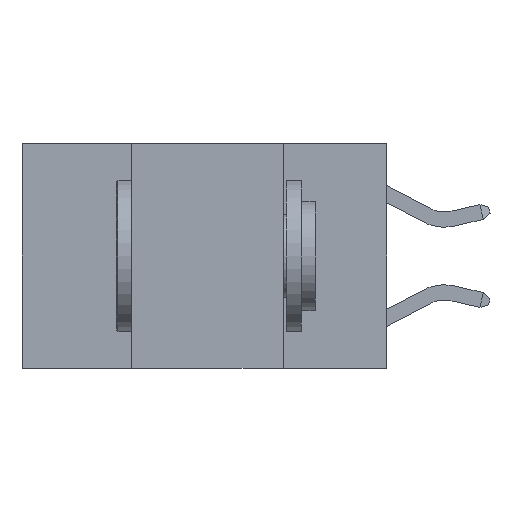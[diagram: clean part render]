
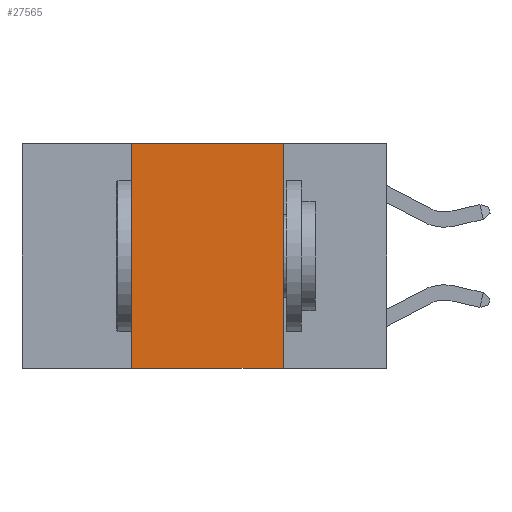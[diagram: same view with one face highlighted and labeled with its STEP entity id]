
A CAD part, left-side view. The second image highlights one B-rep face of the part: STEP entity #27565.
In plain terms, the highlighted planar face has unit normal (-1, 0, 0).
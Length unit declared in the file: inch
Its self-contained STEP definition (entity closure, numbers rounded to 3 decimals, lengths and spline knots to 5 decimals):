
#83 = ORIENTED_EDGE ( 'NONE', *, *, #22307, .F. ) ;
#902 = CARTESIAN_POINT ( 'NONE',  ( 0., 0.6, 0. ) ) ;
#1982 = LINE ( 'NONE', #8722, #28804 ) ;
#2280 = ORIENTED_EDGE ( 'NONE', *, *, #11827, .F. ) ;
#3048 = DIRECTION ( 'NONE',  ( 0., -1., 0. ) ) ;
#3405 = ORIENTED_EDGE ( 'NONE', *, *, #5787, .F. ) ;
#3507 = DIRECTION ( 'NONE',  ( 0., 0., -1. ) ) ;
#3593 = AXIS2_PLACEMENT_3D ( 'NONE', #902, #18667, #3507 ) ;
#5787 = EDGE_CURVE ( 'NONE', #30721, #10411, #27499, .T. ) ;
#8383 = VECTOR ( 'NONE', #12860, 39.37008 ) ;
#8494 = ORIENTED_EDGE ( 'NONE', *, *, #10704, .T. ) ;
#8722 = CARTESIAN_POINT ( 'NONE',  ( 0., 0.6, -0.37 ) ) ;
#9054 = CARTESIAN_POINT ( 'NONE',  ( 0., 0.17, 0. ) ) ;
#10284 = CARTESIAN_POINT ( 'NONE',  ( 0., 0.17, 0. ) ) ;
#10411 = VERTEX_POINT ( 'NONE', #30315 ) ;
#10704 = EDGE_CURVE ( 'NONE', #30721, #30904, #1982, .T. ) ;
#11318 = DIRECTION ( 'NONE',  ( 0., -1., 0. ) ) ;
#11827 = EDGE_CURVE ( 'NONE', #10411, #28912, #27364, .T. ) ;
#12860 = DIRECTION ( 'NONE',  ( 0., 0., -1. ) ) ;
#14054 = VECTOR ( 'NONE', #3048, 39.37008 ) ;
#14245 = CARTESIAN_POINT ( 'NONE',  ( 0., 0.42, 0. ) ) ;
#14987 = VECTOR ( 'NONE', #16797, 39.37008 ) ;
#16797 = DIRECTION ( 'NONE',  ( 0., 0., 1. ) ) ;
#18227 = CARTESIAN_POINT ( 'NONE',  ( 0., 0.6, 0. ) ) ;
#18667 = DIRECTION ( 'NONE',  ( 1., 0., 0. ) ) ;
#19796 = EDGE_LOOP ( 'NONE', ( #83, #2280, #3405, #8494 ) ) ;
#21853 = LINE ( 'NONE', #10284, #8383 ) ;
#22307 = EDGE_CURVE ( 'NONE', #28912, #30904, #21853, .T. ) ;
#22932 = FACE_OUTER_BOUND ( 'NONE', #19796, .T. ) ;
#25660 = CARTESIAN_POINT ( 'NONE',  ( 0., 0.17, -0.37 ) ) ;
#27364 = LINE ( 'NONE', #18227, #14054 ) ;
#27499 = LINE ( 'NONE', #14245, #14987 ) ;
#27565 = ADVANCED_FACE ( 'NONE', ( #22932 ), #31086, .F. ) ;
#28804 = VECTOR ( 'NONE', #11318, 39.37008 ) ;
#28912 = VERTEX_POINT ( 'NONE', #9054 ) ;
#30148 = CARTESIAN_POINT ( 'NONE',  ( 0., 0.42, -0.37 ) ) ;
#30315 = CARTESIAN_POINT ( 'NONE',  ( 0., 0.42, 0. ) ) ;
#30721 = VERTEX_POINT ( 'NONE', #30148 ) ;
#30904 = VERTEX_POINT ( 'NONE', #25660 ) ;
#31086 = PLANE ( 'NONE',  #3593 ) ;
